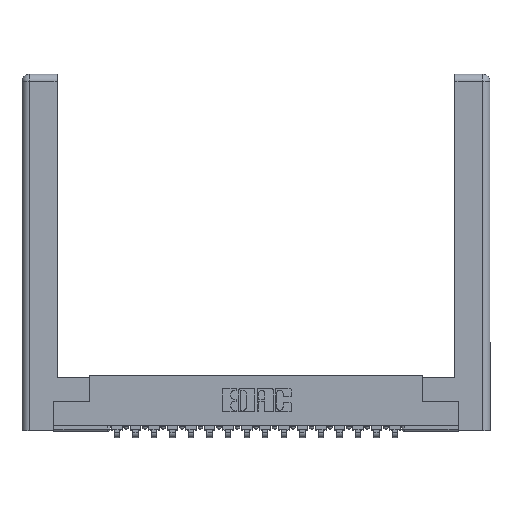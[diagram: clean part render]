
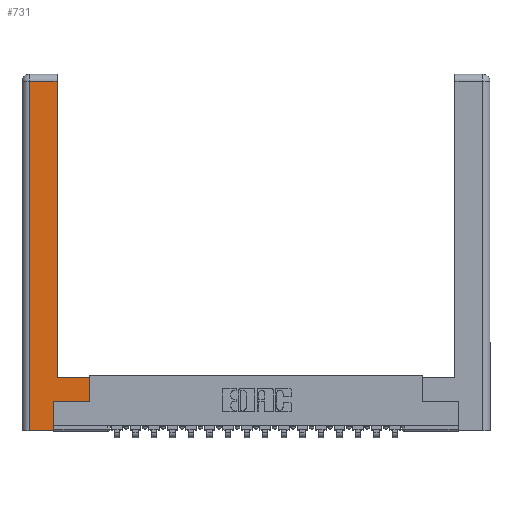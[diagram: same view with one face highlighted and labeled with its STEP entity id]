
A CAD part, top view. The second image highlights one B-rep face of the part: STEP entity #731.
In plain terms, the highlighted planar face has unit normal (0, 0, 1).
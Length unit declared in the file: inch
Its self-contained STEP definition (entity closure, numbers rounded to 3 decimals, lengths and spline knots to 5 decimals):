
#134 = VECTOR ( 'NONE', #14398, 39.37008 ) ;
#234 = DIRECTION ( 'NONE',  ( -1., 0., 0. ) ) ;
#352 = ORIENTED_EDGE ( 'NONE', *, *, #3045, .T. ) ;
#692 = CARTESIAN_POINT ( 'NONE',  ( 0.565, 0.245, 0. ) ) ;
#731 = ADVANCED_FACE ( 'NONE', ( #6579 ), #5038, .F. ) ;
#746 = EDGE_CURVE ( 'NONE', #9781, #2948, #11857, .T. ) ;
#1134 = EDGE_CURVE ( 'NONE', #7549, #12083, #19065, .T. ) ;
#1407 = CARTESIAN_POINT ( 'NONE',  ( 0.265, 0.245, 0. ) ) ;
#1631 = ORIENTED_EDGE ( 'NONE', *, *, #11351, .T. ) ;
#1653 = ORIENTED_EDGE ( 'NONE', *, *, #18818, .T. ) ;
#2203 = ORIENTED_EDGE ( 'NONE', *, *, #11326, .T. ) ;
#2253 = ORIENTED_EDGE ( 'NONE', *, *, #13234, .T. ) ;
#2616 = DIRECTION ( 'NONE',  ( 0., 1., 0. ) ) ;
#2785 = VERTEX_POINT ( 'NONE', #7076 ) ;
#2948 = VERTEX_POINT ( 'NONE', #1407 ) ;
#3045 = EDGE_CURVE ( 'NONE', #4836, #6113, #16055, .T. ) ;
#3577 = LINE ( 'NONE', #692, #13387 ) ;
#3996 = DIRECTION ( 'NONE',  ( 0., 0., -1. ) ) ;
#4045 = CARTESIAN_POINT ( 'NONE',  ( 0.0615, 0., 0. ) ) ;
#4165 = LINE ( 'NONE', #16768, #6490 ) ;
#4303 = DIRECTION ( 'NONE',  ( -1., 0., 0. ) ) ;
#4836 = VERTEX_POINT ( 'NONE', #5087 ) ;
#5038 = PLANE ( 'NONE',  #10694 ) ;
#5087 = CARTESIAN_POINT ( 'NONE',  ( 0.565, 0.45, 0. ) ) ;
#6113 = VERTEX_POINT ( 'NONE', #19137 ) ;
#6318 = LINE ( 'NONE', #20282, #16868 ) ;
#6490 = VECTOR ( 'NONE', #2616, 39.37008 ) ;
#6579 = FACE_OUTER_BOUND ( 'NONE', #18636, .T. ) ;
#7076 = CARTESIAN_POINT ( 'NONE',  ( 0.565, 0.245, 0. ) ) ;
#7549 = VERTEX_POINT ( 'NONE', #11186 ) ;
#7946 = CARTESIAN_POINT ( 'NONE',  ( 0.0615, 0., 0. ) ) ;
#8077 = ORIENTED_EDGE ( 'NONE', *, *, #1134, .T. ) ;
#8906 = VECTOR ( 'NONE', #13244, 39.37008 ) ;
#8937 = DIRECTION ( 'NONE',  ( 0., 1., 0. ) ) ;
#9781 = VERTEX_POINT ( 'NONE', #17670 ) ;
#9822 = CARTESIAN_POINT ( 'NONE',  ( 0.295, 2.94, 0. ) ) ;
#9873 = DIRECTION ( 'NONE',  ( 1., 0., 0. ) ) ;
#10027 = CARTESIAN_POINT ( 'NONE',  ( 0.265, 0., 0. ) ) ;
#10286 = CARTESIAN_POINT ( 'NONE',  ( 0.265, 0.245, 0. ) ) ;
#10694 = AXIS2_PLACEMENT_3D ( 'NONE', #17644, #3996, #4303 ) ;
#11186 = CARTESIAN_POINT ( 'NONE',  ( 0.0615, 2.94, 0. ) ) ;
#11326 = EDGE_CURVE ( 'NONE', #6113, #12161, #17733, .T. ) ;
#11351 = EDGE_CURVE ( 'NONE', #2948, #2785, #3577, .T. ) ;
#11581 = ORIENTED_EDGE ( 'NONE', *, *, #746, .T. ) ;
#11839 = DIRECTION ( 'NONE',  ( 0., 1., 0. ) ) ;
#11857 = LINE ( 'NONE', #10286, #14992 ) ;
#12083 = VERTEX_POINT ( 'NONE', #7946 ) ;
#12161 = VERTEX_POINT ( 'NONE', #9822 ) ;
#13234 = EDGE_CURVE ( 'NONE', #2785, #4836, #4165, .T. ) ;
#13244 = DIRECTION ( 'NONE',  ( 1., 0., 0. ) ) ;
#13387 = VECTOR ( 'NONE', #9873, 39.37008 ) ;
#14398 = DIRECTION ( 'NONE',  ( 0., -1., 0. ) ) ;
#14988 = LINE ( 'NONE', #10027, #8906 ) ;
#14992 = VECTOR ( 'NONE', #8937, 39.37008 ) ;
#16055 = LINE ( 'NONE', #17410, #20137 ) ;
#16659 = ORIENTED_EDGE ( 'NONE', *, *, #17290, .T. ) ;
#16768 = CARTESIAN_POINT ( 'NONE',  ( 0.565, 0.45, 0. ) ) ;
#16868 = VECTOR ( 'NONE', #234, 39.37008 ) ;
#17290 = EDGE_CURVE ( 'NONE', #12083, #9781, #14988, .T. ) ;
#17410 = CARTESIAN_POINT ( 'NONE',  ( 0.295, 0.45, 0. ) ) ;
#17644 = CARTESIAN_POINT ( 'NONE',  ( 0., 0., 0. ) ) ;
#17670 = CARTESIAN_POINT ( 'NONE',  ( 0.265, 0., 0. ) ) ;
#17714 = DIRECTION ( 'NONE',  ( -1., 0., 0. ) ) ;
#17733 = LINE ( 'NONE', #17835, #18982 ) ;
#17835 = CARTESIAN_POINT ( 'NONE',  ( 0.295, 3., 0. ) ) ;
#18636 = EDGE_LOOP ( 'NONE', ( #2203, #1653, #8077, #16659, #11581, #1631, #2253, #352 ) ) ;
#18818 = EDGE_CURVE ( 'NONE', #12161, #7549, #6318, .T. ) ;
#18982 = VECTOR ( 'NONE', #11839, 39.37008 ) ;
#19065 = LINE ( 'NONE', #4045, #134 ) ;
#19137 = CARTESIAN_POINT ( 'NONE',  ( 0.295, 0.45, 0. ) ) ;
#20137 = VECTOR ( 'NONE', #17714, 39.37008 ) ;
#20282 = CARTESIAN_POINT ( 'NONE',  ( 0.0615, 2.94, 0. ) ) ;
